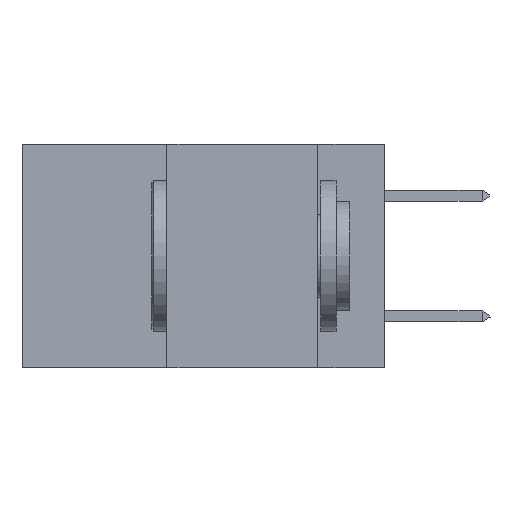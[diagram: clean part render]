
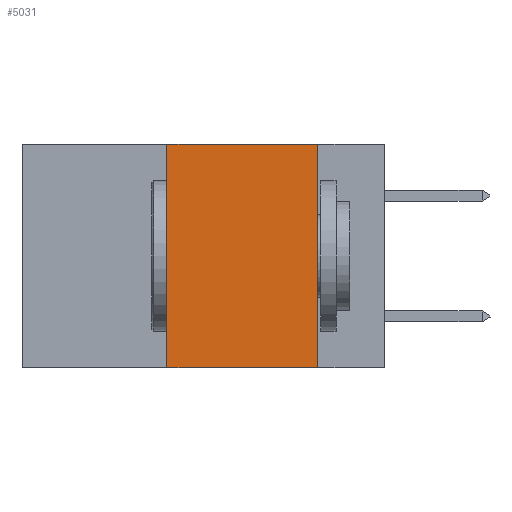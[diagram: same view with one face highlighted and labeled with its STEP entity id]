
A CAD part, left-side view. The second image highlights one B-rep face of the part: STEP entity #5031.
In plain terms, the highlighted planar face has unit normal (-1, 0, 0).
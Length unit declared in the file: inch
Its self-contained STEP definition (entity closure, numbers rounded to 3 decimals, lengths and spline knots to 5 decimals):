
#1197 = VECTOR ( 'NONE', #12800, 39.37008 ) ;
#1206 = CARTESIAN_POINT ( 'NONE',  ( 0., 0.36, 0. ) ) ;
#1273 = ORIENTED_EDGE ( 'NONE', *, *, #11235, .F. ) ;
#1384 = DIRECTION ( 'NONE',  ( 0., 0., -1. ) ) ;
#1694 = VECTOR ( 'NONE', #14959, 39.37008 ) ;
#1912 = CARTESIAN_POINT ( 'NONE',  ( 0., 0.36, -0.37 ) ) ;
#2178 = CARTESIAN_POINT ( 'NONE',  ( 0., 0.11, 0. ) ) ;
#2449 = ORIENTED_EDGE ( 'NONE', *, *, #14547, .F. ) ;
#2741 = FACE_OUTER_BOUND ( 'NONE', #3789, .T. ) ;
#3092 = DIRECTION ( 'NONE',  ( 0., 0., 1. ) ) ;
#3107 = EDGE_CURVE ( 'NONE', #11191, #11940, #11295, .T. ) ;
#3789 = EDGE_LOOP ( 'NONE', ( #6838, #1273, #2449, #13069 ) ) ;
#4588 = DIRECTION ( 'NONE',  ( 0., -1., 0. ) ) ;
#4649 = LINE ( 'NONE', #5125, #1197 ) ;
#5031 = ADVANCED_FACE ( 'NONE', ( #2741 ), #10362, .F. ) ;
#5125 = CARTESIAN_POINT ( 'NONE',  ( 0., 0.6, -0.37 ) ) ;
#6838 = ORIENTED_EDGE ( 'NONE', *, *, #3107, .F. ) ;
#7383 = VECTOR ( 'NONE', #4588, 39.37008 ) ;
#7447 = EDGE_CURVE ( 'NONE', #8079, #11940, #4649, .T. ) ;
#7974 = VERTEX_POINT ( 'NONE', #1206 ) ;
#8079 = VERTEX_POINT ( 'NONE', #1912 ) ;
#8345 = DIRECTION ( 'NONE',  ( 1., 0., 0. ) ) ;
#8877 = CARTESIAN_POINT ( 'NONE',  ( 0., 0.11, 0. ) ) ;
#9345 = CARTESIAN_POINT ( 'NONE',  ( 0., 0.6, 0. ) ) ;
#9746 = VECTOR ( 'NONE', #3092, 39.37008 ) ;
#10014 = CARTESIAN_POINT ( 'NONE',  ( 0., 0.36, 0. ) ) ;
#10362 = PLANE ( 'NONE',  #14292 ) ;
#11058 = CARTESIAN_POINT ( 'NONE',  ( 0., 0.11, -0.37 ) ) ;
#11191 = VERTEX_POINT ( 'NONE', #8877 ) ;
#11235 = EDGE_CURVE ( 'NONE', #7974, #11191, #14407, .T. ) ;
#11295 = LINE ( 'NONE', #2178, #1694 ) ;
#11940 = VERTEX_POINT ( 'NONE', #11058 ) ;
#12523 = CARTESIAN_POINT ( 'NONE',  ( 0., 0.6, 0. ) ) ;
#12800 = DIRECTION ( 'NONE',  ( 0., -1., 0. ) ) ;
#13069 = ORIENTED_EDGE ( 'NONE', *, *, #7447, .T. ) ;
#13322 = LINE ( 'NONE', #10014, #9746 ) ;
#14292 = AXIS2_PLACEMENT_3D ( 'NONE', #9345, #8345, #1384 ) ;
#14407 = LINE ( 'NONE', #12523, #7383 ) ;
#14547 = EDGE_CURVE ( 'NONE', #8079, #7974, #13322, .T. ) ;
#14959 = DIRECTION ( 'NONE',  ( 0., 0., -1. ) ) ;
